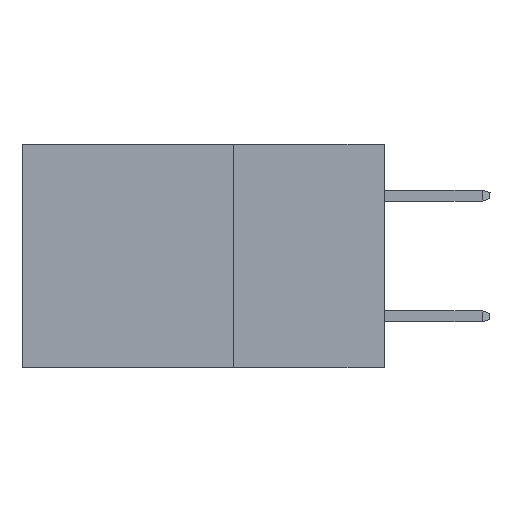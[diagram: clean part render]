
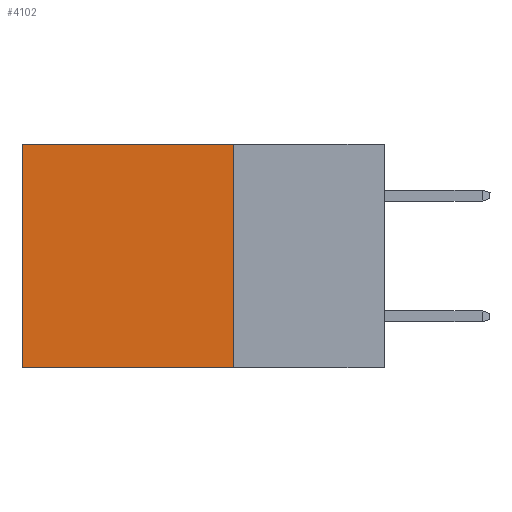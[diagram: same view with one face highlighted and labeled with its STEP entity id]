
A CAD part, left-side view. The second image highlights one B-rep face of the part: STEP entity #4102.
In plain terms, the highlighted planar face has unit normal (-1, 0, 0).
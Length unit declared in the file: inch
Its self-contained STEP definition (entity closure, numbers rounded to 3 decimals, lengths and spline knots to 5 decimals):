
#1942 = LINE ( 'NONE', #27767, #2755 ) ;
#2411 = CARTESIAN_POINT ( 'NONE',  ( 0.298, 0.25, 0. ) ) ;
#2755 = VECTOR ( 'NONE', #4349, 39.37008 ) ;
#4102 = ADVANCED_FACE ( 'NONE', ( #6035 ), #26611, .F. ) ;
#4349 = DIRECTION ( 'NONE',  ( 0., 1., 0. ) ) ;
#5549 = VERTEX_POINT ( 'NONE', #14735 ) ;
#6035 = FACE_OUTER_BOUND ( 'NONE', #23153, .T. ) ;
#6803 = DIRECTION ( 'NONE',  ( 0., 1., 0. ) ) ;
#7342 = CARTESIAN_POINT ( 'NONE',  ( 0.298, 0.25, 0. ) ) ;
#8256 = EDGE_CURVE ( 'NONE', #20844, #33485, #8676, .T. ) ;
#8291 = DIRECTION ( 'NONE',  ( 0., 0., -1. ) ) ;
#8301 = VECTOR ( 'NONE', #33704, 39.37008 ) ;
#8676 = LINE ( 'NONE', #19308, #14813 ) ;
#10471 = DIRECTION ( 'NONE',  ( 1., 0., 0. ) ) ;
#10933 = EDGE_CURVE ( 'NONE', #5549, #33485, #28225, .T. ) ;
#11467 = VERTEX_POINT ( 'NONE', #7342 ) ;
#13050 = DIRECTION ( 'NONE',  ( 0., 0., -1. ) ) ;
#13699 = CARTESIAN_POINT ( 'NONE',  ( 0.298, 0.6, -0.37 ) ) ;
#14735 = CARTESIAN_POINT ( 'NONE',  ( 0.298, 0.6, 0. ) ) ;
#14813 = VECTOR ( 'NONE', #6803, 39.37008 ) ;
#15243 = LINE ( 'NONE', #2411, #8301 ) ;
#15615 = CARTESIAN_POINT ( 'NONE',  ( 0.298, 0.25, -0.37 ) ) ;
#16178 = ORIENTED_EDGE ( 'NONE', *, *, #27141, .T. ) ;
#19308 = CARTESIAN_POINT ( 'NONE',  ( 0.298, 0.25, -0.37 ) ) ;
#19589 = ORIENTED_EDGE ( 'NONE', *, *, #10933, .T. ) ;
#20402 = VECTOR ( 'NONE', #13050, 39.37008 ) ;
#20844 = VERTEX_POINT ( 'NONE', #15615 ) ;
#23153 = EDGE_LOOP ( 'NONE', ( #19589, #27907, #27316, #16178 ) ) ;
#24857 = EDGE_CURVE ( 'NONE', #11467, #20844, #15243, .T. ) ;
#26611 = PLANE ( 'NONE',  #29729 ) ;
#27141 = EDGE_CURVE ( 'NONE', #11467, #5549, #1942, .T. ) ;
#27316 = ORIENTED_EDGE ( 'NONE', *, *, #24857, .F. ) ;
#27767 = CARTESIAN_POINT ( 'NONE',  ( 0.298, 0.25, 0. ) ) ;
#27907 = ORIENTED_EDGE ( 'NONE', *, *, #8256, .F. ) ;
#28225 = LINE ( 'NONE', #31400, #20402 ) ;
#29729 = AXIS2_PLACEMENT_3D ( 'NONE', #32342, #10471, #8291 ) ;
#31400 = CARTESIAN_POINT ( 'NONE',  ( 0.298, 0.6, 0. ) ) ;
#32342 = CARTESIAN_POINT ( 'NONE',  ( 0.298, 0.25, 0. ) ) ;
#33485 = VERTEX_POINT ( 'NONE', #13699 ) ;
#33704 = DIRECTION ( 'NONE',  ( 0., 0., -1. ) ) ;
